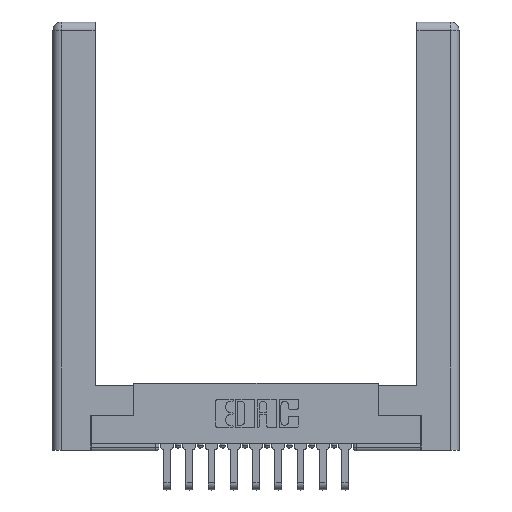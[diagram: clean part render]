
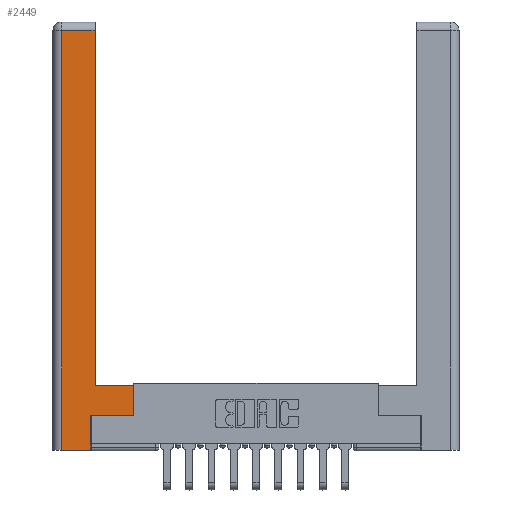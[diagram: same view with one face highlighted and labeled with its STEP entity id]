
A CAD part, top view. The second image highlights one B-rep face of the part: STEP entity #2449.
In plain terms, the highlighted planar face has unit normal (0, 0, 1).
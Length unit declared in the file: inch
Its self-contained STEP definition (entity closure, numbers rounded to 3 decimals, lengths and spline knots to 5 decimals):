
#1057 = LINE ( 'NONE', #7234, #9640 ) ;
#1153 = ORIENTED_EDGE ( 'NONE', *, *, #7532, .T. ) ;
#1285 = DIRECTION ( 'NONE',  ( 0., 0., -1. ) ) ;
#1532 = VERTEX_POINT ( 'NONE', #8497 ) ;
#1559 = DIRECTION ( 'NONE',  ( 0., 1., 0. ) ) ;
#2091 = ORIENTED_EDGE ( 'NONE', *, *, #9145, .T. ) ;
#2131 = VERTEX_POINT ( 'NONE', #7245 ) ;
#2449 = ADVANCED_FACE ( 'NONE', ( #9598 ), #7987, .F. ) ;
#2579 = DIRECTION ( 'NONE',  ( 0., -1., 0. ) ) ;
#3177 = LINE ( 'NONE', #11309, #5458 ) ;
#3291 = ORIENTED_EDGE ( 'NONE', *, *, #14405, .T. ) ;
#3321 = VECTOR ( 'NONE', #2579, 39.37008 ) ;
#3341 = DIRECTION ( 'NONE',  ( -1., 0., 0. ) ) ;
#4481 = DIRECTION ( 'NONE',  ( -1., 0., 0. ) ) ;
#4507 = VERTEX_POINT ( 'NONE', #8759 ) ;
#4548 = VERTEX_POINT ( 'NONE', #8808 ) ;
#4561 = VECTOR ( 'NONE', #12425, 39.37008 ) ;
#4603 = VECTOR ( 'NONE', #5739, 39.37008 ) ;
#4940 = LINE ( 'NONE', #13729, #14417 ) ;
#4990 = ORIENTED_EDGE ( 'NONE', *, *, #10844, .T. ) ;
#5040 = CARTESIAN_POINT ( 'NONE',  ( 0.265, 0., 0. ) ) ;
#5252 = ORIENTED_EDGE ( 'NONE', *, *, #6513, .T. ) ;
#5458 = VECTOR ( 'NONE', #3341, 39.37008 ) ;
#5739 = DIRECTION ( 'NONE',  ( 0., 1., 0. ) ) ;
#5788 = CARTESIAN_POINT ( 'NONE',  ( 0.265, 0.245, 0. ) ) ;
#6296 = LINE ( 'NONE', #12680, #3321 ) ;
#6316 = LINE ( 'NONE', #5040, #7910 ) ;
#6322 = AXIS2_PLACEMENT_3D ( 'NONE', #9034, #1285, #4481 ) ;
#6355 = EDGE_CURVE ( 'NONE', #12412, #11695, #6861, .T. ) ;
#6399 = VECTOR ( 'NONE', #8984, 39.37008 ) ;
#6513 = EDGE_CURVE ( 'NONE', #7149, #2131, #6316, .T. ) ;
#6550 = CARTESIAN_POINT ( 'NONE',  ( 0.0615, 0., 0. ) ) ;
#6861 = LINE ( 'NONE', #7918, #4561 ) ;
#7149 = VERTEX_POINT ( 'NONE', #6550 ) ;
#7234 = CARTESIAN_POINT ( 'NONE',  ( 0.295, 3., 0. ) ) ;
#7245 = CARTESIAN_POINT ( 'NONE',  ( 0.265, 0., 0. ) ) ;
#7532 = EDGE_CURVE ( 'NONE', #4548, #12412, #1057, .T. ) ;
#7539 = CARTESIAN_POINT ( 'NONE',  ( 0.295, 2.94, 0. ) ) ;
#7910 = VECTOR ( 'NONE', #10446, 39.37008 ) ;
#7918 = CARTESIAN_POINT ( 'NONE',  ( 0.0615, 2.94, 0. ) ) ;
#7987 = PLANE ( 'NONE',  #6322 ) ;
#8133 = DIRECTION ( 'NONE',  ( 0., 1., 0. ) ) ;
#8497 = CARTESIAN_POINT ( 'NONE',  ( 0.265, 0.245, 0. ) ) ;
#8658 = CARTESIAN_POINT ( 'NONE',  ( 0.0615, 2.94, 0. ) ) ;
#8714 = LINE ( 'NONE', #11173, #6399 ) ;
#8759 = CARTESIAN_POINT ( 'NONE',  ( 0.565, 0.245, 0. ) ) ;
#8808 = CARTESIAN_POINT ( 'NONE',  ( 0.295, 0.45, 0. ) ) ;
#8984 = DIRECTION ( 'NONE',  ( 1., 0., 0. ) ) ;
#9034 = CARTESIAN_POINT ( 'NONE',  ( 0., 0., 0. ) ) ;
#9145 = EDGE_CURVE ( 'NONE', #1532, #4507, #8714, .T. ) ;
#9224 = CARTESIAN_POINT ( 'NONE',  ( 0.565, 0.45, 0. ) ) ;
#9400 = ORIENTED_EDGE ( 'NONE', *, *, #11993, .T. ) ;
#9598 = FACE_OUTER_BOUND ( 'NONE', #12732, .T. ) ;
#9640 = VECTOR ( 'NONE', #1559, 39.37008 ) ;
#10231 = LINE ( 'NONE', #5788, #4603 ) ;
#10446 = DIRECTION ( 'NONE',  ( 1., 0., 0. ) ) ;
#10844 = EDGE_CURVE ( 'NONE', #2131, #1532, #10231, .T. ) ;
#11173 = CARTESIAN_POINT ( 'NONE',  ( 0.565, 0.245, 0. ) ) ;
#11309 = CARTESIAN_POINT ( 'NONE',  ( 0.295, 0.45, 0. ) ) ;
#11361 = ORIENTED_EDGE ( 'NONE', *, *, #11566, .T. ) ;
#11566 = EDGE_CURVE ( 'NONE', #4507, #14456, #4940, .T. ) ;
#11695 = VERTEX_POINT ( 'NONE', #8658 ) ;
#11993 = EDGE_CURVE ( 'NONE', #14456, #4548, #3177, .T. ) ;
#12412 = VERTEX_POINT ( 'NONE', #7539 ) ;
#12425 = DIRECTION ( 'NONE',  ( -1., 0., 0. ) ) ;
#12445 = ORIENTED_EDGE ( 'NONE', *, *, #6355, .T. ) ;
#12680 = CARTESIAN_POINT ( 'NONE',  ( 0.0615, 0., 0. ) ) ;
#12732 = EDGE_LOOP ( 'NONE', ( #1153, #12445, #3291, #5252, #4990, #2091, #11361, #9400 ) ) ;
#13729 = CARTESIAN_POINT ( 'NONE',  ( 0.565, 0.45, 0. ) ) ;
#14405 = EDGE_CURVE ( 'NONE', #11695, #7149, #6296, .T. ) ;
#14417 = VECTOR ( 'NONE', #8133, 39.37008 ) ;
#14456 = VERTEX_POINT ( 'NONE', #9224 ) ;
